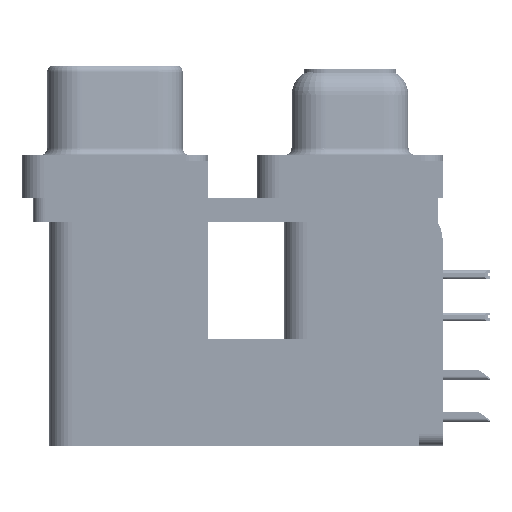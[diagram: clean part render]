
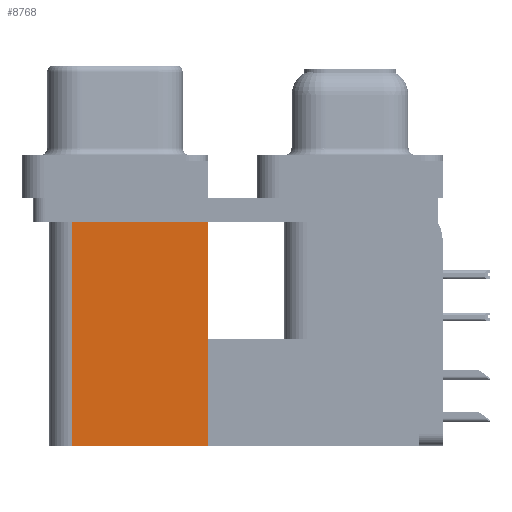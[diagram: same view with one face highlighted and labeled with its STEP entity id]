
A CAD part, left-side view. The second image highlights one B-rep face of the part: STEP entity #8768.
In plain terms, the highlighted planar face has unit normal (-1, 0, 0).
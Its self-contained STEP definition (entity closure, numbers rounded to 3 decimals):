
#392 = VECTOR ( 'NONE', #48135, 1000. ) ;
#515 = EDGE_CURVE ( 'NONE', #15219, #53330, #19463, .T. ) ;
#1808 = LINE ( 'NONE', #14319, #392 ) ;
#2584 = CARTESIAN_POINT ( 'NONE',  ( 3.7, 9.6, -2.5 ) ) ;
#2860 = DIRECTION ( 'NONE',  ( 0., 0., 1. ) ) ;
#3741 = DIRECTION ( 'NONE',  ( 0., 0., -1. ) ) ;
#4082 = LINE ( 'NONE', #16592, #41399 ) ;
#7642 = FACE_OUTER_BOUND ( 'NONE', #31217, .T. ) ;
#8768 = ADVANCED_FACE ( 'NONE', ( #7642 ), #12365, .F. ) ;
#11200 = CARTESIAN_POINT ( 'NONE',  ( 3.7, 9.6, -19.2 ) ) ;
#11811 = CARTESIAN_POINT ( 'NONE',  ( 3.7, 9.6, -19.2 ) ) ;
#12365 = PLANE ( 'NONE',  #32035 ) ;
#12532 = VECTOR ( 'NONE', #14210, 1000. ) ;
#12977 = ORIENTED_EDGE ( 'NONE', *, *, #44083, .F. ) ;
#14210 = DIRECTION ( 'NONE',  ( 0., 0., 1. ) ) ;
#14317 = EDGE_CURVE ( 'NONE', #27039, #18700, #31739, .T. ) ;
#14319 = CARTESIAN_POINT ( 'NONE',  ( 3.7, 9.6, -19.2 ) ) ;
#14484 = CARTESIAN_POINT ( 'NONE',  ( 3.7, 18.8, -19.2 ) ) ;
#15219 = VERTEX_POINT ( 'NONE', #33702 ) ;
#16592 = CARTESIAN_POINT ( 'NONE',  ( 3.7, 9.6, -2.5 ) ) ;
#18700 = VERTEX_POINT ( 'NONE', #2584 ) ;
#19270 = EDGE_CURVE ( 'NONE', #18700, #53330, #4082, .T. ) ;
#19463 = LINE ( 'NONE', #14484, #12532 ) ;
#25447 = DIRECTION ( 'NONE',  ( 0., 1., 0. ) ) ;
#27039 = VERTEX_POINT ( 'NONE', #46495 ) ;
#27112 = ORIENTED_EDGE ( 'NONE', *, *, #19270, .T. ) ;
#31217 = EDGE_LOOP ( 'NONE', ( #27112, #51276, #12977, #51873 ) ) ;
#31739 = LINE ( 'NONE', #11200, #48228 ) ;
#32035 = AXIS2_PLACEMENT_3D ( 'NONE', #11811, #45637, #3741 ) ;
#33702 = CARTESIAN_POINT ( 'NONE',  ( 3.7, 18.8, -19.2 ) ) ;
#37396 = CARTESIAN_POINT ( 'NONE',  ( 3.7, 18.8, -2.5 ) ) ;
#41399 = VECTOR ( 'NONE', #25447, 1000. ) ;
#44083 = EDGE_CURVE ( 'NONE', #27039, #15219, #1808, .T. ) ;
#45637 = DIRECTION ( 'NONE',  ( 1., 0., 0. ) ) ;
#46495 = CARTESIAN_POINT ( 'NONE',  ( 3.7, 9.6, -19.2 ) ) ;
#48135 = DIRECTION ( 'NONE',  ( 0., 1., 0. ) ) ;
#48228 = VECTOR ( 'NONE', #2860, 1000. ) ;
#51276 = ORIENTED_EDGE ( 'NONE', *, *, #515, .F. ) ;
#51873 = ORIENTED_EDGE ( 'NONE', *, *, #14317, .T. ) ;
#53330 = VERTEX_POINT ( 'NONE', #37396 ) ;
